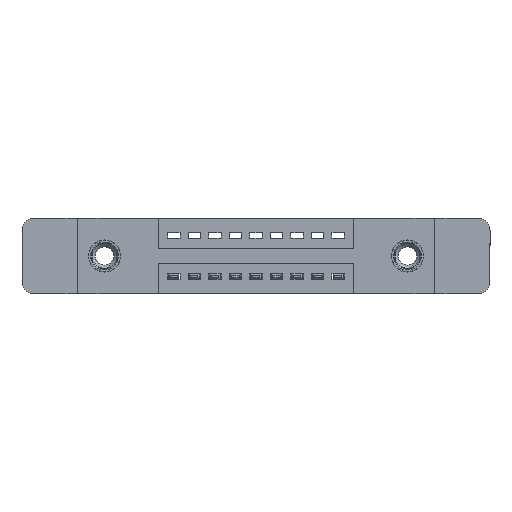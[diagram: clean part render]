
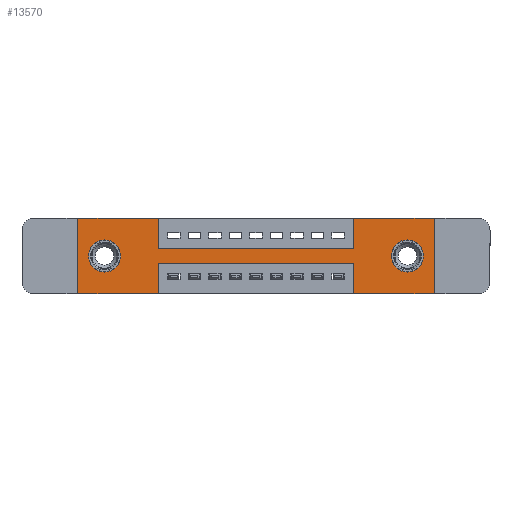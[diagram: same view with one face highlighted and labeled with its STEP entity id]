
A CAD part, front view. The second image highlights one B-rep face of the part: STEP entity #13570.
In plain terms, the highlighted planar face has unit normal (0, -1, 0).
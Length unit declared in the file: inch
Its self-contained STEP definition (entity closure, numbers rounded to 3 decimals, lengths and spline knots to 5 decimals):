
#32 = CARTESIAN_POINT ( 'NONE',  ( 0., 0., 0. ) ) ;
#82 = VECTOR ( 'NONE', #3535, 39.37008 ) ;
#108 = CARTESIAN_POINT ( 'NONE',  ( 1.605, 0., -0.185 ) ) ;
#125 = VERTEX_POINT ( 'NONE', #799 ) ;
#230 = CIRCLE ( 'NONE', #4566, 0.078 ) ;
#299 = ORIENTED_EDGE ( 'NONE', *, *, #5570, .F. ) ;
#300 = VERTEX_POINT ( 'NONE', #2713 ) ;
#721 = LINE ( 'NONE', #12647, #6797 ) ;
#747 = CARTESIAN_POINT ( 'NONE',  ( 0.13, 0., -0.107 ) ) ;
#799 = CARTESIAN_POINT ( 'NONE',  ( 1.735, 0., 0. ) ) ;
#989 = DIRECTION ( 'NONE',  ( 0., 0., -1. ) ) ;
#1030 = VERTEX_POINT ( 'NONE', #9918 ) ;
#1315 = ORIENTED_EDGE ( 'NONE', *, *, #11204, .T. ) ;
#1645 = ORIENTED_EDGE ( 'NONE', *, *, #10593, .F. ) ;
#1809 = VECTOR ( 'NONE', #3092, 39.37008 ) ;
#1857 = DIRECTION ( 'NONE',  ( 0., 0., 1. ) ) ;
#2087 = VECTOR ( 'NONE', #2122, 39.37008 ) ;
#2122 = DIRECTION ( 'NONE',  ( 0., 0., -1. ) ) ;
#2273 = ORIENTED_EDGE ( 'NONE', *, *, #5266, .T. ) ;
#2322 = ORIENTED_EDGE ( 'NONE', *, *, #14886, .F. ) ;
#2423 = CARTESIAN_POINT ( 'NONE',  ( 0.3925, 0., 0. ) ) ;
#2519 = EDGE_CURVE ( 'NONE', #7374, #6234, #5880, .T. ) ;
#2614 = LINE ( 'NONE', #13192, #1809 ) ;
#2691 = LINE ( 'NONE', #10366, #12068 ) ;
#2713 = CARTESIAN_POINT ( 'NONE',  ( 0.3925, 0., 0. ) ) ;
#2748 = CARTESIAN_POINT ( 'NONE',  ( 0., 0., -0.37 ) ) ;
#3092 = DIRECTION ( 'NONE',  ( 0., 0., -1. ) ) ;
#3157 = VECTOR ( 'NONE', #10197, 39.37008 ) ;
#3185 = CARTESIAN_POINT ( 'NONE',  ( 0.13, 0., -0.185 ) ) ;
#3333 = DIRECTION ( 'NONE',  ( 0., 0., -1. ) ) ;
#3535 = DIRECTION ( 'NONE',  ( 0., 0., 1. ) ) ;
#3663 = VERTEX_POINT ( 'NONE', #747 ) ;
#3699 = DIRECTION ( 'NONE',  ( 0., -1., 0. ) ) ;
#3792 = EDGE_CURVE ( 'NONE', #15336, #3806, #14572, .T. ) ;
#3806 = VERTEX_POINT ( 'NONE', #14801 ) ;
#4328 = LINE ( 'NONE', #2748, #15093 ) ;
#4414 = LINE ( 'NONE', #13100, #12802 ) ;
#4487 = AXIS2_PLACEMENT_3D ( 'NONE', #8339, #9710, #15913 ) ;
#4566 = AXIS2_PLACEMENT_3D ( 'NONE', #13296, #4610, #14525 ) ;
#4610 = DIRECTION ( 'NONE',  ( 0., 1., 0. ) ) ;
#4794 = ORIENTED_EDGE ( 'NONE', *, *, #13429, .T. ) ;
#4861 = VECTOR ( 'NONE', #11249, 39.37008 ) ;
#4975 = CARTESIAN_POINT ( 'NONE',  ( 0.3925, 0., -0.22 ) ) ;
#5109 = DIRECTION ( 'NONE',  ( 0., 0., 1. ) ) ;
#5266 = EDGE_CURVE ( 'NONE', #8185, #3663, #13753, .T. ) ;
#5289 = DIRECTION ( 'NONE',  ( -1., 0., 0. ) ) ;
#5293 = CARTESIAN_POINT ( 'NONE',  ( 0., 0., 0. ) ) ;
#5570 = EDGE_CURVE ( 'NONE', #300, #8039, #8832, .T. ) ;
#5880 = LINE ( 'NONE', #7618, #12117 ) ;
#5928 = VECTOR ( 'NONE', #989, 39.37008 ) ;
#6015 = CIRCLE ( 'NONE', #6281, 0.078 ) ;
#6234 = VERTEX_POINT ( 'NONE', #4975 ) ;
#6243 = ORIENTED_EDGE ( 'NONE', *, *, #11995, .F. ) ;
#6245 = FACE_BOUND ( 'NONE', #13333, .T. ) ;
#6281 = AXIS2_PLACEMENT_3D ( 'NONE', #108, #9081, #3333 ) ;
#6551 = VERTEX_POINT ( 'NONE', #8687 ) ;
#6608 = CARTESIAN_POINT ( 'NONE',  ( 0.3925, 0., -0.37 ) ) ;
#6645 = ORIENTED_EDGE ( 'NONE', *, *, #9019, .F. ) ;
#6758 = VERTEX_POINT ( 'NONE', #8464 ) ;
#6797 = VECTOR ( 'NONE', #5109, 39.37008 ) ;
#7032 = FACE_OUTER_BOUND ( 'NONE', #14680, .T. ) ;
#7162 = ORIENTED_EDGE ( 'NONE', *, *, #12652, .F. ) ;
#7374 = VERTEX_POINT ( 'NONE', #14716 ) ;
#7527 = DIRECTION ( 'NONE',  ( 0., 0., -1. ) ) ;
#7618 = CARTESIAN_POINT ( 'NONE',  ( 0.3925, 0., -0.22 ) ) ;
#7619 = VECTOR ( 'NONE', #5289, 39.37008 ) ;
#7802 = CARTESIAN_POINT ( 'NONE',  ( 1.735, 0., -0.37 ) ) ;
#8039 = VERTEX_POINT ( 'NONE', #15170 ) ;
#8067 = DIRECTION ( 'NONE',  ( 1., 0., 0. ) ) ;
#8160 = CARTESIAN_POINT ( 'NONE',  ( 1.605, 0., -0.263 ) ) ;
#8185 = VERTEX_POINT ( 'NONE', #13885 ) ;
#8234 = CARTESIAN_POINT ( 'NONE',  ( 0.3925, 0., -0.37 ) ) ;
#8339 = CARTESIAN_POINT ( 'NONE',  ( 1.605, 0., -0.185 ) ) ;
#8341 = EDGE_LOOP ( 'NONE', ( #1315, #2273 ) ) ;
#8363 = VERTEX_POINT ( 'NONE', #6608 ) ;
#8464 = CARTESIAN_POINT ( 'NONE',  ( 0., 0., -0.37 ) ) ;
#8604 = EDGE_CURVE ( 'NONE', #13854, #1030, #6015, .T. ) ;
#8667 = CARTESIAN_POINT ( 'NONE',  ( 1.3425, 0., -0.37 ) ) ;
#8687 = CARTESIAN_POINT ( 'NONE',  ( 1.3425, 0., -0.37 ) ) ;
#8773 = EDGE_CURVE ( 'NONE', #6234, #8363, #11079, .T. ) ;
#8823 = PLANE ( 'NONE',  #13901 ) ;
#8832 = LINE ( 'NONE', #2423, #5928 ) ;
#9019 = EDGE_CURVE ( 'NONE', #6758, #13076, #721, .T. ) ;
#9072 = DIRECTION ( 'NONE',  ( -1., 0., 0. ) ) ;
#9081 = DIRECTION ( 'NONE',  ( 0., 1., 0. ) ) ;
#9294 = DIRECTION ( 'NONE',  ( 0., 1., 0. ) ) ;
#9710 = DIRECTION ( 'NONE',  ( 0., 1., 0. ) ) ;
#9830 = CARTESIAN_POINT ( 'NONE',  ( 1.3425, 0., 0. ) ) ;
#9891 = VERTEX_POINT ( 'NONE', #7802 ) ;
#9918 = CARTESIAN_POINT ( 'NONE',  ( 1.605, 0., -0.107 ) ) ;
#9958 = EDGE_CURVE ( 'NONE', #3806, #125, #4414, .T. ) ;
#10197 = DIRECTION ( 'NONE',  ( 1., 0., 0. ) ) ;
#10366 = CARTESIAN_POINT ( 'NONE',  ( 0.3925, 0., -0.15 ) ) ;
#10593 = EDGE_CURVE ( 'NONE', #125, #9891, #2614, .T. ) ;
#10863 = ORIENTED_EDGE ( 'NONE', *, *, #9958, .F. ) ;
#11079 = LINE ( 'NONE', #8234, #2087 ) ;
#11107 = ORIENTED_EDGE ( 'NONE', *, *, #3792, .F. ) ;
#11204 = EDGE_CURVE ( 'NONE', #3663, #8185, #230, .T. ) ;
#11249 = DIRECTION ( 'NONE',  ( 0., 0., 1. ) ) ;
#11521 = ORIENTED_EDGE ( 'NONE', *, *, #14672, .F. ) ;
#11534 = DIRECTION ( 'NONE',  ( -1., 0., 0. ) ) ;
#11995 = EDGE_CURVE ( 'NONE', #13076, #300, #12146, .T. ) ;
#12068 = VECTOR ( 'NONE', #8067, 39.37008 ) ;
#12117 = VECTOR ( 'NONE', #9072, 39.37008 ) ;
#12146 = LINE ( 'NONE', #5293, #3157 ) ;
#12170 = ORIENTED_EDGE ( 'NONE', *, *, #8773, .F. ) ;
#12647 = CARTESIAN_POINT ( 'NONE',  ( 0., 0., 0. ) ) ;
#12652 = EDGE_CURVE ( 'NONE', #8363, #6758, #4328, .T. ) ;
#12692 = ORIENTED_EDGE ( 'NONE', *, *, #13682, .F. ) ;
#12802 = VECTOR ( 'NONE', #12986, 39.37008 ) ;
#12986 = DIRECTION ( 'NONE',  ( 1., 0., 0. ) ) ;
#13076 = VERTEX_POINT ( 'NONE', #32 ) ;
#13100 = CARTESIAN_POINT ( 'NONE',  ( 0., 0., 0. ) ) ;
#13192 = CARTESIAN_POINT ( 'NONE',  ( 1.735, 0., 0. ) ) ;
#13198 = AXIS2_PLACEMENT_3D ( 'NONE', #3185, #9294, #1857 ) ;
#13296 = CARTESIAN_POINT ( 'NONE',  ( 0.13, 0., -0.185 ) ) ;
#13333 = EDGE_LOOP ( 'NONE', ( #4794, #15311 ) ) ;
#13429 = EDGE_CURVE ( 'NONE', #1030, #13854, #16056, .T. ) ;
#13570 = ADVANCED_FACE ( 'NONE', ( #6245, #13690, #7032 ), #8823, .T. ) ;
#13682 = EDGE_CURVE ( 'NONE', #9891, #6551, #15454, .T. ) ;
#13690 = FACE_BOUND ( 'NONE', #8341, .T. ) ;
#13753 = CIRCLE ( 'NONE', #13198, 0.078 ) ;
#13854 = VERTEX_POINT ( 'NONE', #8160 ) ;
#13885 = CARTESIAN_POINT ( 'NONE',  ( 0.13, 0., -0.263 ) ) ;
#13901 = AXIS2_PLACEMENT_3D ( 'NONE', #15072, #3699, #7527 ) ;
#14013 = CARTESIAN_POINT ( 'NONE',  ( 0., 0., -0.37 ) ) ;
#14525 = DIRECTION ( 'NONE',  ( 0., 0., 1. ) ) ;
#14572 = LINE ( 'NONE', #9830, #82 ) ;
#14618 = LINE ( 'NONE', #8667, #4861 ) ;
#14672 = EDGE_CURVE ( 'NONE', #6551, #7374, #14618, .T. ) ;
#14680 = EDGE_LOOP ( 'NONE', ( #12170, #14906, #11521, #12692, #1645, #10863, #11107, #2322, #299, #6243, #6645, #7162 ) ) ;
#14716 = CARTESIAN_POINT ( 'NONE',  ( 1.3425, 0., -0.22 ) ) ;
#14801 = CARTESIAN_POINT ( 'NONE',  ( 1.3425, 0., 0. ) ) ;
#14886 = EDGE_CURVE ( 'NONE', #8039, #15336, #2691, .T. ) ;
#14888 = CARTESIAN_POINT ( 'NONE',  ( 1.3425, 0., -0.15 ) ) ;
#14906 = ORIENTED_EDGE ( 'NONE', *, *, #2519, .F. ) ;
#15072 = CARTESIAN_POINT ( 'NONE',  ( 0., 0., -0.37 ) ) ;
#15093 = VECTOR ( 'NONE', #11534, 39.37008 ) ;
#15170 = CARTESIAN_POINT ( 'NONE',  ( 0.3925, 0., -0.15 ) ) ;
#15311 = ORIENTED_EDGE ( 'NONE', *, *, #8604, .T. ) ;
#15336 = VERTEX_POINT ( 'NONE', #14888 ) ;
#15454 = LINE ( 'NONE', #14013, #7619 ) ;
#15913 = DIRECTION ( 'NONE',  ( 0., 0., -1. ) ) ;
#16056 = CIRCLE ( 'NONE', #4487, 0.078 ) ;
